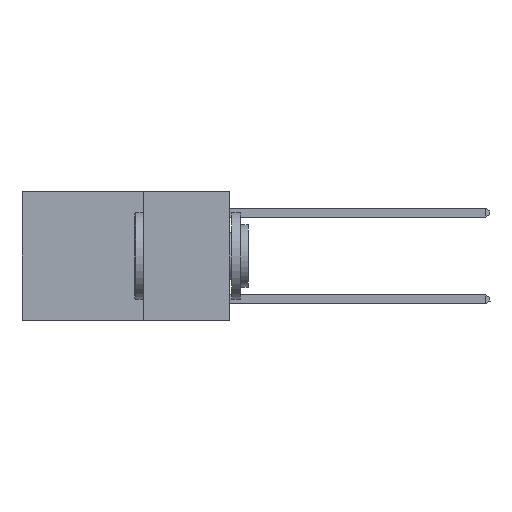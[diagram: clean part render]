
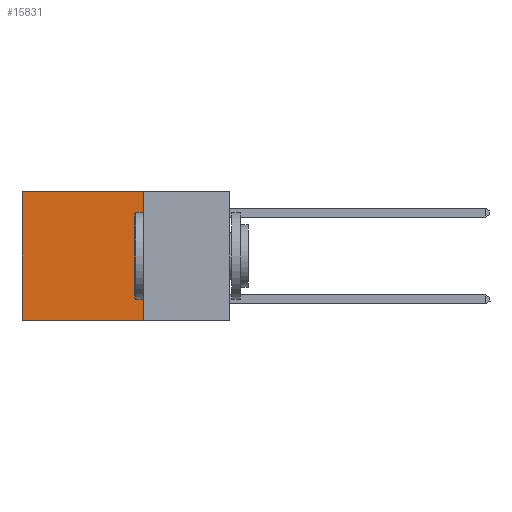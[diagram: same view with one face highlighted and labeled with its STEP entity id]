
A CAD part, left-side view. The second image highlights one B-rep face of the part: STEP entity #15831.
In plain terms, the highlighted planar face has unit normal (-1, 0, 0).
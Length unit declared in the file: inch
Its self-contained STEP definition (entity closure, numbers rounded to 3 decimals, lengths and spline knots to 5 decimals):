
#485 = FACE_OUTER_BOUND ( 'NONE', #25246, .T. ) ;
#497 = DIRECTION ( 'NONE',  ( 0., 0., -1. ) ) ;
#1233 = VECTOR ( 'NONE', #19788, 39.37008 ) ;
#2491 = VECTOR ( 'NONE', #497, 39.37008 ) ;
#2899 = CARTESIAN_POINT ( 'NONE',  ( 0.2625, 0.25, -0.37 ) ) ;
#3076 = VERTEX_POINT ( 'NONE', #22690 ) ;
#3149 = CARTESIAN_POINT ( 'NONE',  ( 0.2625, 0.25, 0. ) ) ;
#4468 = VERTEX_POINT ( 'NONE', #11450 ) ;
#4899 = DIRECTION ( 'NONE',  ( 0., 0., -1. ) ) ;
#5588 = DIRECTION ( 'NONE',  ( 0., 1., 0. ) ) ;
#5777 = ORIENTED_EDGE ( 'NONE', *, *, #12952, .F. ) ;
#7465 = CARTESIAN_POINT ( 'NONE',  ( 0.2625, 0.25, 0. ) ) ;
#7503 = CARTESIAN_POINT ( 'NONE',  ( 0.2625, 0.25, 0. ) ) ;
#7566 = DIRECTION ( 'NONE',  ( 1., 0., 0. ) ) ;
#7739 = DIRECTION ( 'NONE',  ( 0., 0., -1. ) ) ;
#8619 = VERTEX_POINT ( 'NONE', #7465 ) ;
#11053 = CARTESIAN_POINT ( 'NONE',  ( 0.2625, 0.25, -0.37 ) ) ;
#11450 = CARTESIAN_POINT ( 'NONE',  ( 0.2625, 0.6, -0.37 ) ) ;
#11495 = VECTOR ( 'NONE', #5588, 39.37008 ) ;
#11565 = PLANE ( 'NONE',  #25079 ) ;
#12023 = CARTESIAN_POINT ( 'NONE',  ( 0.2625, 0.6, 0. ) ) ;
#12057 = VERTEX_POINT ( 'NONE', #11053 ) ;
#12952 = EDGE_CURVE ( 'NONE', #12057, #4468, #22884, .T. ) ;
#13238 = EDGE_CURVE ( 'NONE', #8619, #3076, #17120, .T. ) ;
#14118 = EDGE_CURVE ( 'NONE', #8619, #12057, #27477, .T. ) ;
#14996 = VECTOR ( 'NONE', #7739, 39.37008 ) ;
#15104 = ORIENTED_EDGE ( 'NONE', *, *, #13238, .T. ) ;
#15831 = ADVANCED_FACE ( 'NONE', ( #485 ), #11565, .F. ) ;
#16927 = EDGE_CURVE ( 'NONE', #3076, #4468, #20749, .T. ) ;
#17120 = LINE ( 'NONE', #7503, #11495 ) ;
#17459 = CARTESIAN_POINT ( 'NONE',  ( 0.2625, 0.25, 0. ) ) ;
#19150 = ORIENTED_EDGE ( 'NONE', *, *, #14118, .F. ) ;
#19788 = DIRECTION ( 'NONE',  ( 0., 1., 0. ) ) ;
#20749 = LINE ( 'NONE', #12023, #14996 ) ;
#22690 = CARTESIAN_POINT ( 'NONE',  ( 0.2625, 0.6, 0. ) ) ;
#22884 = LINE ( 'NONE', #2899, #1233 ) ;
#25079 = AXIS2_PLACEMENT_3D ( 'NONE', #3149, #7566, #4899 ) ;
#25246 = EDGE_LOOP ( 'NONE', ( #26297, #5777, #19150, #15104 ) ) ;
#26297 = ORIENTED_EDGE ( 'NONE', *, *, #16927, .T. ) ;
#27477 = LINE ( 'NONE', #17459, #2491 ) ;
